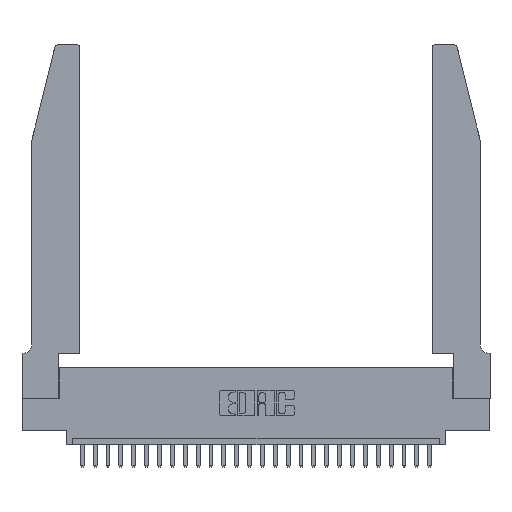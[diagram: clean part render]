
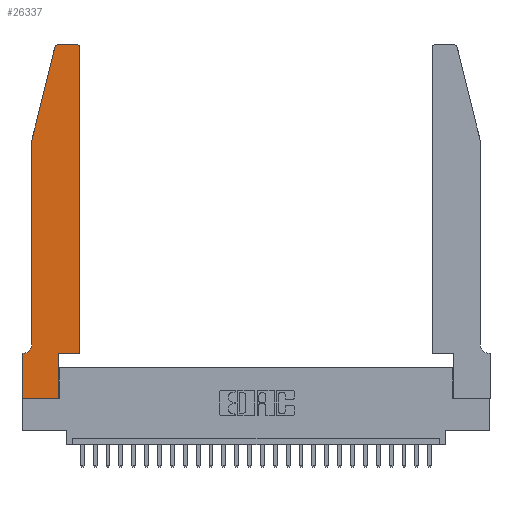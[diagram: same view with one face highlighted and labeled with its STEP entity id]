
A CAD part, top view. The second image highlights one B-rep face of the part: STEP entity #26337.
In plain terms, the highlighted planar face has unit normal (0, 0, 1).
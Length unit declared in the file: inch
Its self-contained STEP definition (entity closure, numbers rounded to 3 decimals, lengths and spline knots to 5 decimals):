
#753 = CARTESIAN_POINT ( 'NONE',  ( 0.0755, 0.42, 0.37 ) ) ;
#914 = CIRCLE ( 'NONE', #4165, 0.03 ) ;
#1364 = VECTOR ( 'NONE', #18540, 39.37008 ) ;
#1449 = ORIENTED_EDGE ( 'NONE', *, *, #9292, .T. ) ;
#1478 = LINE ( 'NONE', #2312, #25830 ) ;
#1803 = ORIENTED_EDGE ( 'NONE', *, *, #4868, .T. ) ;
#1890 = DIRECTION ( 'NONE',  ( 1., 0., 0. ) ) ;
#2312 = CARTESIAN_POINT ( 'NONE',  ( 0.4505, 0.35, 0.37 ) ) ;
#3125 = EDGE_LOOP ( 'NONE', ( #13705, #19414, #16618, #9451, #21185, #20040, #27761, #26389, #1449, #11503, #1803, #24128 ) ) ;
#3223 = VERTEX_POINT ( 'NONE', #9326 ) ;
#3273 = CARTESIAN_POINT ( 'NONE',  ( 0.2865, 0., 0.37 ) ) ;
#3710 = CARTESIAN_POINT ( 'NONE',  ( 0.4205, 2.75, 0.37 ) ) ;
#4165 = AXIS2_PLACEMENT_3D ( 'NONE', #21135, #12722, #25602 ) ;
#4868 = EDGE_CURVE ( 'NONE', #15850, #8121, #1478, .T. ) ;
#5049 = VERTEX_POINT ( 'NONE', #753 ) ;
#5677 = DIRECTION ( 'NONE',  ( 0., -1., 0. ) ) ;
#5755 = VECTOR ( 'NONE', #6083, 39.37008 ) ;
#5784 = LINE ( 'NONE', #20613, #25434 ) ;
#5974 = CARTESIAN_POINT ( 'NONE',  ( 0., 0., 0.37 ) ) ;
#6057 = CARTESIAN_POINT ( 'NONE',  ( 0.4505, 0.35, 0.37 ) ) ;
#6083 = DIRECTION ( 'NONE',  ( 1., 0., 0. ) ) ;
#6625 = DIRECTION ( 'NONE',  ( 0., 0., -1. ) ) ;
#6914 = VERTEX_POINT ( 'NONE', #7666 ) ;
#7150 = VERTEX_POINT ( 'NONE', #3273 ) ;
#7666 = CARTESIAN_POINT ( 'NONE',  ( 0.0755, 2., 0.37 ) ) ;
#8121 = VERTEX_POINT ( 'NONE', #23247 ) ;
#8394 = EDGE_CURVE ( 'NONE', #8949, #25381, #5784, .T. ) ;
#8949 = VERTEX_POINT ( 'NONE', #12137 ) ;
#9104 = CARTESIAN_POINT ( 'NONE',  ( 0.0755, 0.35, 0.37 ) ) ;
#9292 = EDGE_CURVE ( 'NONE', #7150, #25942, #11159, .T. ) ;
#9326 = CARTESIAN_POINT ( 'NONE',  ( 0.284, 2.75, 0.37 ) ) ;
#9451 = ORIENTED_EDGE ( 'NONE', *, *, #21481, .T. ) ;
#10295 = DIRECTION ( 'NONE',  ( 0., 1., 0. ) ) ;
#10365 = DIRECTION ( 'NONE',  ( 1., 0., 0. ) ) ;
#10491 = LINE ( 'NONE', #9104, #1364 ) ;
#10925 = CARTESIAN_POINT ( 'NONE',  ( 0.0055, 0.42, 0.37 ) ) ;
#11072 = EDGE_CURVE ( 'NONE', #8121, #27320, #14102, .T. ) ;
#11142 = EDGE_CURVE ( 'NONE', #12274, #6914, #15446, .T. ) ;
#11159 = LINE ( 'NONE', #26642, #20960 ) ;
#11503 = ORIENTED_EDGE ( 'NONE', *, *, #15275, .T. ) ;
#12137 = CARTESIAN_POINT ( 'NONE',  ( 0., 0.35, 0.37 ) ) ;
#12274 = VERTEX_POINT ( 'NONE', #20799 ) ;
#12722 = DIRECTION ( 'NONE',  ( 0., 0., 1. ) ) ;
#13120 = DIRECTION ( 'NONE',  ( 1., 0., 0. ) ) ;
#13434 = DIRECTION ( 'NONE',  ( -1., 0., 0. ) ) ;
#13485 = CARTESIAN_POINT ( 'NONE',  ( 0.0755, 2., 0.37 ) ) ;
#13620 = DIRECTION ( 'NONE',  ( -1., 0., 0. ) ) ;
#13651 = VECTOR ( 'NONE', #10365, 39.37008 ) ;
#13705 = ORIENTED_EDGE ( 'NONE', *, *, #26996, .T. ) ;
#14102 = CIRCLE ( 'NONE', #27093, 0.03 ) ;
#15026 = CARTESIAN_POINT ( 'NONE',  ( 0.4205, 2.72, 0.37 ) ) ;
#15275 = EDGE_CURVE ( 'NONE', #25942, #15850, #15918, .T. ) ;
#15446 = LINE ( 'NONE', #13485, #27939 ) ;
#15850 = VERTEX_POINT ( 'NONE', #6057 ) ;
#15918 = LINE ( 'NONE', #21407, #5755 ) ;
#16608 = DIRECTION ( 'NONE',  ( 0., 1., 0. ) ) ;
#16618 = ORIENTED_EDGE ( 'NONE', *, *, #11142, .T. ) ;
#17213 = DIRECTION ( 'NONE',  ( 0., 0., 1. ) ) ;
#17776 = DIRECTION ( 'NONE',  ( -0.239, -0.971, 0. ) ) ;
#18245 = LINE ( 'NONE', #20289, #24682 ) ;
#18272 = EDGE_CURVE ( 'NONE', #5049, #25224, #21864, .T. ) ;
#18475 = AXIS2_PLACEMENT_3D ( 'NONE', #10925, #6625, #13434 ) ;
#18540 = DIRECTION ( 'NONE',  ( -1., 0., 0. ) ) ;
#18962 = PLANE ( 'NONE',  #20769 ) ;
#19414 = ORIENTED_EDGE ( 'NONE', *, *, #27734, .T. ) ;
#19555 = VECTOR ( 'NONE', #13620, 39.37008 ) ;
#19557 = CARTESIAN_POINT ( 'NONE',  ( 0.2865, 0.35, 0.37 ) ) ;
#19938 = EDGE_CURVE ( 'NONE', #25381, #7150, #20073, .T. ) ;
#20040 = ORIENTED_EDGE ( 'NONE', *, *, #25477, .T. ) ;
#20073 = LINE ( 'NONE', #5974, #13651 ) ;
#20289 = CARTESIAN_POINT ( 'NONE',  ( 0.0755, 2., 0.37 ) ) ;
#20613 = CARTESIAN_POINT ( 'NONE',  ( 0., 0., 0.37 ) ) ;
#20769 = AXIS2_PLACEMENT_3D ( 'NONE', #27652, #25319, #1890 ) ;
#20799 = CARTESIAN_POINT ( 'NONE',  ( 0.25487, 2.72718, 0.37 ) ) ;
#20960 = VECTOR ( 'NONE', #10295, 39.37008 ) ;
#21089 = CARTESIAN_POINT ( 'NONE',  ( 0.2605, 2.75, 0.37 ) ) ;
#21135 = CARTESIAN_POINT ( 'NONE',  ( 0.284, 2.72, 0.37 ) ) ;
#21185 = ORIENTED_EDGE ( 'NONE', *, *, #18272, .T. ) ;
#21407 = CARTESIAN_POINT ( 'NONE',  ( 0.4505, 0.35, 0.37 ) ) ;
#21481 = EDGE_CURVE ( 'NONE', #6914, #5049, #18245, .T. ) ;
#21864 = CIRCLE ( 'NONE', #18475, 0.07 ) ;
#23247 = CARTESIAN_POINT ( 'NONE',  ( 0.4505, 2.72, 0.37 ) ) ;
#23605 = LINE ( 'NONE', #21089, #19555 ) ;
#24128 = ORIENTED_EDGE ( 'NONE', *, *, #11072, .T. ) ;
#24682 = VECTOR ( 'NONE', #27023, 39.37008 ) ;
#25224 = VERTEX_POINT ( 'NONE', #27904 ) ;
#25319 = DIRECTION ( 'NONE',  ( 0., 0., 1. ) ) ;
#25381 = VERTEX_POINT ( 'NONE', #26216 ) ;
#25434 = VECTOR ( 'NONE', #5677, 39.37008 ) ;
#25477 = EDGE_CURVE ( 'NONE', #25224, #8949, #10491, .T. ) ;
#25602 = DIRECTION ( 'NONE',  ( 1., 0., 0. ) ) ;
#25830 = VECTOR ( 'NONE', #16608, 39.37008 ) ;
#25942 = VERTEX_POINT ( 'NONE', #19557 ) ;
#26216 = CARTESIAN_POINT ( 'NONE',  ( 0., 0., 0.37 ) ) ;
#26315 = FACE_OUTER_BOUND ( 'NONE', #3125, .T. ) ;
#26337 = ADVANCED_FACE ( 'NONE', ( #26315 ), #18962, .T. ) ;
#26389 = ORIENTED_EDGE ( 'NONE', *, *, #19938, .T. ) ;
#26642 = CARTESIAN_POINT ( 'NONE',  ( 0.2865, 0.35, 0.37 ) ) ;
#26996 = EDGE_CURVE ( 'NONE', #27320, #3223, #23605, .T. ) ;
#27023 = DIRECTION ( 'NONE',  ( 0., -1., 0. ) ) ;
#27093 = AXIS2_PLACEMENT_3D ( 'NONE', #15026, #17213, #13120 ) ;
#27320 = VERTEX_POINT ( 'NONE', #3710 ) ;
#27652 = CARTESIAN_POINT ( 'NONE',  ( 0., 0.35, 0.37 ) ) ;
#27734 = EDGE_CURVE ( 'NONE', #3223, #12274, #914, .T. ) ;
#27761 = ORIENTED_EDGE ( 'NONE', *, *, #8394, .T. ) ;
#27904 = CARTESIAN_POINT ( 'NONE',  ( 0.0055, 0.35, 0.37 ) ) ;
#27939 = VECTOR ( 'NONE', #17776, 39.37008 ) ;
